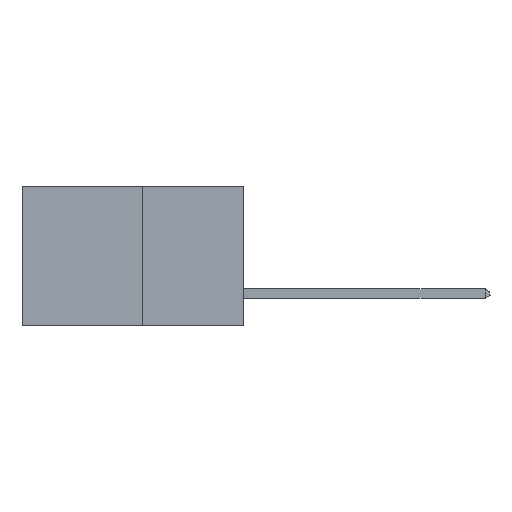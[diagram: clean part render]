
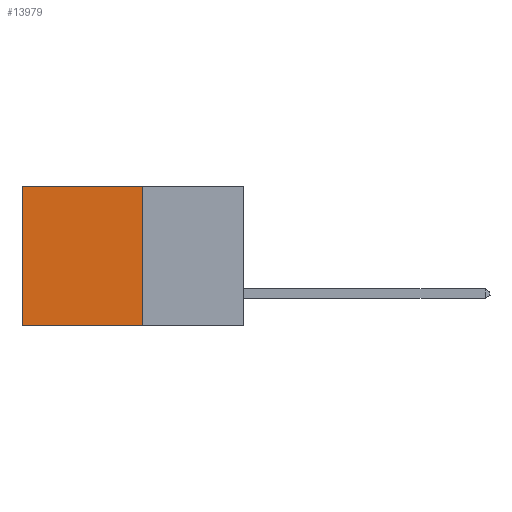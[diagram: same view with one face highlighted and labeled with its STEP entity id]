
A CAD part, left-side view. The second image highlights one B-rep face of the part: STEP entity #13979.
In plain terms, the highlighted planar face has unit normal (-1, 0, 0).
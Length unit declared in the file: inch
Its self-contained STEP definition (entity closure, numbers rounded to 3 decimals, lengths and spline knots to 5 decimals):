
#88 = DIRECTION ( 'NONE',  ( 1., 0., 0. ) ) ;
#1274 = VECTOR ( 'NONE', #15370, 39.37008 ) ;
#1650 = EDGE_CURVE ( 'NONE', #29518, #8502, #2848, .T. ) ;
#2848 = LINE ( 'NONE', #11314, #8387 ) ;
#2958 = ORIENTED_EDGE ( 'NONE', *, *, #1650, .T. ) ;
#3593 = CARTESIAN_POINT ( 'NONE',  ( 0.277, 0.59, 0. ) ) ;
#5696 = CARTESIAN_POINT ( 'NONE',  ( 0.277, 0.27, -0.37 ) ) ;
#6281 = DIRECTION ( 'NONE',  ( 0., 0., -1. ) ) ;
#6848 = FACE_OUTER_BOUND ( 'NONE', #28127, .T. ) ;
#8387 = VECTOR ( 'NONE', #6281, 39.37008 ) ;
#8502 = VERTEX_POINT ( 'NONE', #28236 ) ;
#8609 = DIRECTION ( 'NONE',  ( 0., 1., 0. ) ) ;
#9699 = VERTEX_POINT ( 'NONE', #15118 ) ;
#11314 = CARTESIAN_POINT ( 'NONE',  ( 0.277, 0.59, -0.37 ) ) ;
#11417 = VERTEX_POINT ( 'NONE', #21382 ) ;
#12334 = ORIENTED_EDGE ( 'NONE', *, *, #12527, .T. ) ;
#12527 = EDGE_CURVE ( 'NONE', #9699, #29518, #18347, .T. ) ;
#12681 = CARTESIAN_POINT ( 'NONE',  ( 0.277, 0.27, -0.37 ) ) ;
#13117 = EDGE_CURVE ( 'NONE', #9699, #11417, #13866, .T. ) ;
#13866 = LINE ( 'NONE', #29418, #1274 ) ;
#13979 = ADVANCED_FACE ( 'NONE', ( #6848 ), #14270, .F. ) ;
#14270 = PLANE ( 'NONE',  #28096 ) ;
#15118 = CARTESIAN_POINT ( 'NONE',  ( 0.277, 0.27, 0. ) ) ;
#15370 = DIRECTION ( 'NONE',  ( 0., 0., -1. ) ) ;
#15452 = ORIENTED_EDGE ( 'NONE', *, *, #28950, .F. ) ;
#16685 = DIRECTION ( 'NONE',  ( 0., 0., -1. ) ) ;
#18042 = VECTOR ( 'NONE', #24527, 39.37008 ) ;
#18347 = LINE ( 'NONE', #20304, #26119 ) ;
#20304 = CARTESIAN_POINT ( 'NONE',  ( 0.277, 0.27, 0. ) ) ;
#21382 = CARTESIAN_POINT ( 'NONE',  ( 0.277, 0.27, -0.37 ) ) ;
#23561 = LINE ( 'NONE', #5696, #18042 ) ;
#24527 = DIRECTION ( 'NONE',  ( 0., 1., 0. ) ) ;
#26119 = VECTOR ( 'NONE', #8609, 39.37008 ) ;
#27116 = ORIENTED_EDGE ( 'NONE', *, *, #13117, .F. ) ;
#28096 = AXIS2_PLACEMENT_3D ( 'NONE', #12681, #88, #16685 ) ;
#28127 = EDGE_LOOP ( 'NONE', ( #2958, #15452, #27116, #12334 ) ) ;
#28236 = CARTESIAN_POINT ( 'NONE',  ( 0.277, 0.59, -0.37 ) ) ;
#28950 = EDGE_CURVE ( 'NONE', #11417, #8502, #23561, .T. ) ;
#29418 = CARTESIAN_POINT ( 'NONE',  ( 0.277, 0.27, -0.37 ) ) ;
#29518 = VERTEX_POINT ( 'NONE', #3593 ) ;
